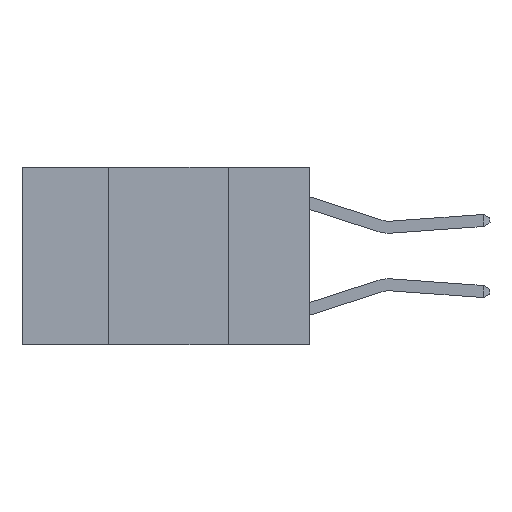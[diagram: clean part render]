
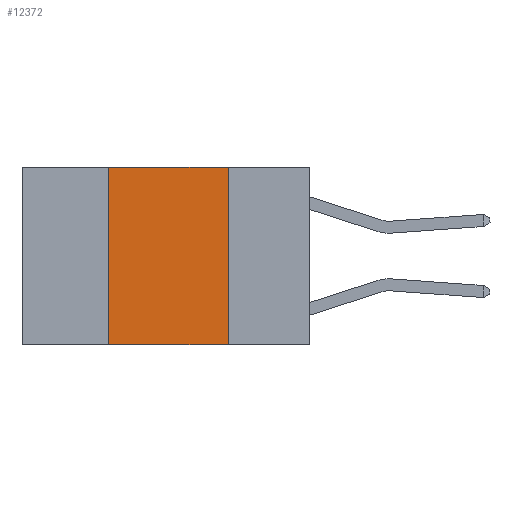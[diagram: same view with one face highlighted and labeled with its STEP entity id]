
A CAD part, left-side view. The second image highlights one B-rep face of the part: STEP entity #12372.
In plain terms, the highlighted planar face has unit normal (-1, 0, 0).
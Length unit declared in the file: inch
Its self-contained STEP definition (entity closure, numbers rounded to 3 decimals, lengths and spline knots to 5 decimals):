
#919 = CARTESIAN_POINT ( 'NONE',  ( 0., 0.17, -0.37 ) ) ;
#2720 = VECTOR ( 'NONE', #6247, 39.37008 ) ;
#3454 = VERTEX_POINT ( 'NONE', #27279 ) ;
#3664 = PLANE ( 'NONE',  #24131 ) ;
#4376 = VERTEX_POINT ( 'NONE', #919 ) ;
#6247 = DIRECTION ( 'NONE',  ( 0., 0., 1. ) ) ;
#6603 = CARTESIAN_POINT ( 'NONE',  ( 0., 0.6, 0. ) ) ;
#7964 = DIRECTION ( 'NONE',  ( 1., 0., 0. ) ) ;
#8648 = ORIENTED_EDGE ( 'NONE', *, *, #26374, .T. ) ;
#9206 = VERTEX_POINT ( 'NONE', #17440 ) ;
#9242 = CARTESIAN_POINT ( 'NONE',  ( 0., 0.17, 0. ) ) ;
#11423 = EDGE_CURVE ( 'NONE', #9206, #18892, #18109, .T. ) ;
#11531 = ORIENTED_EDGE ( 'NONE', *, *, #18863, .F. ) ;
#12372 = ADVANCED_FACE ( 'NONE', ( #13124 ), #3664, .F. ) ;
#12422 = EDGE_LOOP ( 'NONE', ( #19081, #15170, #11531, #8648 ) ) ;
#13124 = FACE_OUTER_BOUND ( 'NONE', #12422, .T. ) ;
#13306 = CARTESIAN_POINT ( 'NONE',  ( 0., 0.6, -0.37 ) ) ;
#14708 = LINE ( 'NONE', #13306, #24525 ) ;
#15125 = LINE ( 'NONE', #9242, #26853 ) ;
#15170 = ORIENTED_EDGE ( 'NONE', *, *, #11423, .F. ) ;
#15431 = DIRECTION ( 'NONE',  ( 0., -1., 0. ) ) ;
#17440 = CARTESIAN_POINT ( 'NONE',  ( 0., 0.42, 0. ) ) ;
#18109 = LINE ( 'NONE', #6603, #22347 ) ;
#18498 = CARTESIAN_POINT ( 'NONE',  ( 0., 0.6, 0. ) ) ;
#18863 = EDGE_CURVE ( 'NONE', #3454, #9206, #20270, .T. ) ;
#18892 = VERTEX_POINT ( 'NONE', #25209 ) ;
#19081 = ORIENTED_EDGE ( 'NONE', *, *, #24473, .F. ) ;
#20270 = LINE ( 'NONE', #25117, #2720 ) ;
#22347 = VECTOR ( 'NONE', #23736, 39.37008 ) ;
#22685 = DIRECTION ( 'NONE',  ( 0., 0., -1. ) ) ;
#23736 = DIRECTION ( 'NONE',  ( 0., -1., 0. ) ) ;
#24131 = AXIS2_PLACEMENT_3D ( 'NONE', #18498, #7964, #22685 ) ;
#24473 = EDGE_CURVE ( 'NONE', #18892, #4376, #15125, .T. ) ;
#24525 = VECTOR ( 'NONE', #15431, 39.37008 ) ;
#25117 = CARTESIAN_POINT ( 'NONE',  ( 0., 0.42, 0. ) ) ;
#25209 = CARTESIAN_POINT ( 'NONE',  ( 0., 0.17, 0. ) ) ;
#25950 = DIRECTION ( 'NONE',  ( 0., 0., -1. ) ) ;
#26374 = EDGE_CURVE ( 'NONE', #3454, #4376, #14708, .T. ) ;
#26853 = VECTOR ( 'NONE', #25950, 39.37008 ) ;
#27279 = CARTESIAN_POINT ( 'NONE',  ( 0., 0.42, -0.37 ) ) ;
